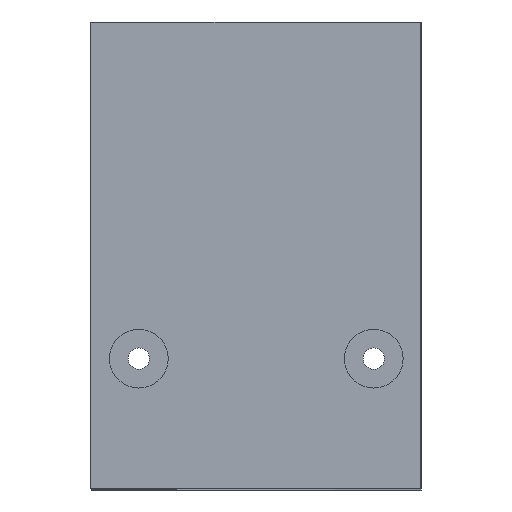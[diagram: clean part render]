
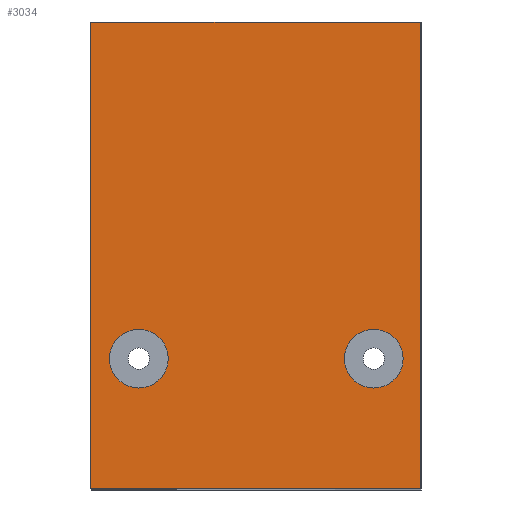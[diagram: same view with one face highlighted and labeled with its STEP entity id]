
A CAD part, front view. The second image highlights one B-rep face of the part: STEP entity #3034.
In plain terms, the highlighted planar face has unit normal (0, -1, 0).
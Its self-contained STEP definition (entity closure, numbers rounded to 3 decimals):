
#532 = PLANE('',#533);
#533 = AXIS2_PLACEMENT_3D('',#534,#535,#536);
#534 = CARTESIAN_POINT('',(76.2,22.676,20.811));
#535 = DIRECTION('',(0.,0.,-1.));
#536 = DIRECTION('',(0.,1.,0.));
#1657 = VERTEX_POINT('',#1658);
#1658 = CARTESIAN_POINT('',(76.103,23.345,20.811));
#1672 = PLANE('',#1673);
#1673 = AXIS2_PLACEMENT_3D('',#1674,#1675,#1676);
#1674 = CARTESIAN_POINT('',(76.103,42.545,-31.631));
#1675 = DIRECTION('',(-1.,0.,0.));
#1676 = DIRECTION('',(0.,0.,1.));
#1684 = EDGE_CURVE('',#1657,#1685,#1687,.T.);
#1685 = VERTEX_POINT('',#1686);
#1686 = CARTESIAN_POINT('',(39.094,23.345,20.811));
#1687 = SURFACE_CURVE('',#1688,(#1692,#1699),.PCURVE_S1.);
#1688 = LINE('',#1689,#1690);
#1689 = CARTESIAN_POINT('',(76.151,23.345,20.811));
#1690 = VECTOR('',#1691,1.);
#1691 = DIRECTION('',(-1.,0.,0.));
#1692 = PCURVE('',#532,#1693);
#1693 = DEFINITIONAL_REPRESENTATION('',(#1694),#1698);
#1694 = LINE('',#1695,#1696);
#1695 = CARTESIAN_POINT('',(0.669,-0.049));
#1696 = VECTOR('',#1697,1.);
#1697 = DIRECTION('',(0.,-1.));
#1698 = ( GEOMETRIC_REPRESENTATION_CONTEXT(2) 
PARAMETRIC_REPRESENTATION_CONTEXT() REPRESENTATION_CONTEXT('2D SPACE',''
  ) );
#1699 = PCURVE('',#1700,#1705);
#1700 = PLANE('',#1701);
#1701 = AXIS2_PLACEMENT_3D('',#1702,#1703,#1704);
#1702 = CARTESIAN_POINT('',(76.103,23.345,20.829));
#1703 = DIRECTION('',(0.,1.,0.));
#1704 = DIRECTION('',(0.,0.,1.));
#1705 = DEFINITIONAL_REPRESENTATION('',(#1706),#1710);
#1706 = LINE('',#1707,#1708);
#1707 = CARTESIAN_POINT('',(-0.018,0.049));
#1708 = VECTOR('',#1709,1.);
#1709 = DIRECTION('',(0.,-1.));
#1710 = ( GEOMETRIC_REPRESENTATION_CONTEXT(2) 
PARAMETRIC_REPRESENTATION_CONTEXT() REPRESENTATION_CONTEXT('2D SPACE',''
  ) );
#1726 = PLANE('',#1727);
#1727 = AXIS2_PLACEMENT_3D('',#1728,#1729,#1730);
#1728 = CARTESIAN_POINT('',(39.094,42.545,20.829));
#1729 = DIRECTION('',(1.,0.,0.));
#1730 = DIRECTION('',(0.,0.,-1.));
#1897 = PLANE('',#1898);
#1898 = AXIS2_PLACEMENT_3D('',#1899,#1900,#1901);
#1899 = CARTESIAN_POINT('',(39.094,42.545,-31.631));
#1900 = DIRECTION('',(0.,0.,1.));
#1901 = DIRECTION('',(1.,0.,0.));
#2990 = EDGE_CURVE('',#1685,#2991,#2993,.T.);
#2991 = VERTEX_POINT('',#2992);
#2992 = CARTESIAN_POINT('',(39.094,23.345,-31.631));
#2993 = SURFACE_CURVE('',#2994,(#2998,#3005),.PCURVE_S1.);
#2994 = LINE('',#2995,#2996);
#2995 = CARTESIAN_POINT('',(39.094,23.345,20.829));
#2996 = VECTOR('',#2997,1.);
#2997 = DIRECTION('',(0.,0.,-1.));
#2998 = PCURVE('',#1726,#2999);
#2999 = DEFINITIONAL_REPRESENTATION('',(#3000),#3004);
#3000 = LINE('',#3001,#3002);
#3001 = CARTESIAN_POINT('',(0.,-19.2));
#3002 = VECTOR('',#3003,1.);
#3003 = DIRECTION('',(1.,0.));
#3004 = ( GEOMETRIC_REPRESENTATION_CONTEXT(2) 
PARAMETRIC_REPRESENTATION_CONTEXT() REPRESENTATION_CONTEXT('2D SPACE',''
  ) );
#3005 = PCURVE('',#1700,#3006);
#3006 = DEFINITIONAL_REPRESENTATION('',(#3007),#3011);
#3007 = LINE('',#3008,#3009);
#3008 = CARTESIAN_POINT('',(0.,-37.009));
#3009 = VECTOR('',#3010,1.);
#3010 = DIRECTION('',(-1.,0.));
#3011 = ( GEOMETRIC_REPRESENTATION_CONTEXT(2) 
PARAMETRIC_REPRESENTATION_CONTEXT() REPRESENTATION_CONTEXT('2D SPACE',''
  ) );
#3034 = ADVANCED_FACE('',(#3035,#3083,#3118),#1700,.F.);
#3035 = FACE_BOUND('',#3036,.F.);
#3036 = EDGE_LOOP('',(#3037,#3038,#3061,#3082));
#3037 = ORIENTED_EDGE('',*,*,#1684,.F.);
#3038 = ORIENTED_EDGE('',*,*,#3039,.F.);
#3039 = EDGE_CURVE('',#3040,#1657,#3042,.T.);
#3040 = VERTEX_POINT('',#3041);
#3041 = CARTESIAN_POINT('',(76.103,23.345,-31.631));
#3042 = SURFACE_CURVE('',#3043,(#3047,#3054),.PCURVE_S1.);
#3043 = LINE('',#3044,#3045);
#3044 = CARTESIAN_POINT('',(76.103,23.345,-31.631));
#3045 = VECTOR('',#3046,1.);
#3046 = DIRECTION('',(0.,0.,1.));
#3047 = PCURVE('',#1700,#3048);
#3048 = DEFINITIONAL_REPRESENTATION('',(#3049),#3053);
#3049 = LINE('',#3050,#3051);
#3050 = CARTESIAN_POINT('',(-52.459,0.));
#3051 = VECTOR('',#3052,1.);
#3052 = DIRECTION('',(1.,0.));
#3053 = ( GEOMETRIC_REPRESENTATION_CONTEXT(2) 
PARAMETRIC_REPRESENTATION_CONTEXT() REPRESENTATION_CONTEXT('2D SPACE',''
  ) );
#3054 = PCURVE('',#1672,#3055);
#3055 = DEFINITIONAL_REPRESENTATION('',(#3056),#3060);
#3056 = LINE('',#3057,#3058);
#3057 = CARTESIAN_POINT('',(0.,-19.2));
#3058 = VECTOR('',#3059,1.);
#3059 = DIRECTION('',(1.,0.));
#3060 = ( GEOMETRIC_REPRESENTATION_CONTEXT(2) 
PARAMETRIC_REPRESENTATION_CONTEXT() REPRESENTATION_CONTEXT('2D SPACE',''
  ) );
#3061 = ORIENTED_EDGE('',*,*,#3062,.F.);
#3062 = EDGE_CURVE('',#2991,#3040,#3063,.T.);
#3063 = SURFACE_CURVE('',#3064,(#3068,#3075),.PCURVE_S1.);
#3064 = LINE('',#3065,#3066);
#3065 = CARTESIAN_POINT('',(39.094,23.345,-31.631));
#3066 = VECTOR('',#3067,1.);
#3067 = DIRECTION('',(1.,0.,0.));
#3068 = PCURVE('',#1700,#3069);
#3069 = DEFINITIONAL_REPRESENTATION('',(#3070),#3074);
#3070 = LINE('',#3071,#3072);
#3071 = CARTESIAN_POINT('',(-52.459,-37.009));
#3072 = VECTOR('',#3073,1.);
#3073 = DIRECTION('',(0.,1.));
#3074 = ( GEOMETRIC_REPRESENTATION_CONTEXT(2) 
PARAMETRIC_REPRESENTATION_CONTEXT() REPRESENTATION_CONTEXT('2D SPACE',''
  ) );
#3075 = PCURVE('',#1897,#3076);
#3076 = DEFINITIONAL_REPRESENTATION('',(#3077),#3081);
#3077 = LINE('',#3078,#3079);
#3078 = CARTESIAN_POINT('',(0.,-19.2));
#3079 = VECTOR('',#3080,1.);
#3080 = DIRECTION('',(1.,0.));
#3081 = ( GEOMETRIC_REPRESENTATION_CONTEXT(2) 
PARAMETRIC_REPRESENTATION_CONTEXT() REPRESENTATION_CONTEXT('2D SPACE',''
  ) );
#3082 = ORIENTED_EDGE('',*,*,#2990,.F.);
#3083 = FACE_BOUND('',#3084,.F.);
#3084 = EDGE_LOOP('',(#3085));
#3085 = ORIENTED_EDGE('',*,*,#3086,.T.);
#3086 = EDGE_CURVE('',#3087,#3087,#3089,.T.);
#3087 = VERTEX_POINT('',#3088);
#3088 = CARTESIAN_POINT('',(47.792,23.345,-17.));
#3089 = SURFACE_CURVE('',#3090,(#3095,#3106),.PCURVE_S1.);
#3090 = CIRCLE('',#3091,3.3);
#3091 = AXIS2_PLACEMENT_3D('',#3092,#3093,#3094);
#3092 = CARTESIAN_POINT('',(44.492,23.345,-17.));
#3093 = DIRECTION('',(0.,-1.,0.));
#3094 = DIRECTION('',(1.,0.,0.));
#3095 = PCURVE('',#1700,#3096);
#3096 = DEFINITIONAL_REPRESENTATION('',(#3097),#3105);
#3097 = ( BOUNDED_CURVE() B_SPLINE_CURVE(2,(#3098,#3099,#3100,#3101,
#3102,#3103,#3104),.UNSPECIFIED.,.T.,.F.) B_SPLINE_CURVE_WITH_KNOTS((1,2
    ,2,2,2,1),(-2.094,0.,2.094,4.189,
6.283,8.378),.UNSPECIFIED.) CURVE() 
GEOMETRIC_REPRESENTATION_ITEM() RATIONAL_B_SPLINE_CURVE((1.,0.5,1.,0.5,
1.,0.5,1.)) REPRESENTATION_ITEM('') );
#3098 = CARTESIAN_POINT('',(-37.829,-28.31));
#3099 = CARTESIAN_POINT('',(-32.113,-28.31));
#3100 = CARTESIAN_POINT('',(-34.971,-33.26));
#3101 = CARTESIAN_POINT('',(-37.829,-38.21));
#3102 = CARTESIAN_POINT('',(-40.686,-33.26));
#3103 = CARTESIAN_POINT('',(-43.544,-28.31));
#3104 = CARTESIAN_POINT('',(-37.829,-28.31));
#3105 = ( GEOMETRIC_REPRESENTATION_CONTEXT(2) 
PARAMETRIC_REPRESENTATION_CONTEXT() REPRESENTATION_CONTEXT('2D SPACE',''
  ) );
#3106 = PCURVE('',#3107,#3112);
#3107 = CYLINDRICAL_SURFACE('',#3108,3.3);
#3108 = AXIS2_PLACEMENT_3D('',#3109,#3110,#3111);
#3109 = CARTESIAN_POINT('',(44.492,23.345,-17.));
#3110 = DIRECTION('',(0.,-1.,0.));
#3111 = DIRECTION('',(1.,0.,0.));
#3112 = DEFINITIONAL_REPRESENTATION('',(#3113),#3117);
#3113 = LINE('',#3114,#3115);
#3114 = CARTESIAN_POINT('',(0.,0.));
#3115 = VECTOR('',#3116,1.);
#3116 = DIRECTION('',(1.,0.));
#3117 = ( GEOMETRIC_REPRESENTATION_CONTEXT(2) 
PARAMETRIC_REPRESENTATION_CONTEXT() REPRESENTATION_CONTEXT('2D SPACE',''
  ) );
#3118 = FACE_BOUND('',#3119,.F.);
#3119 = EDGE_LOOP('',(#3120));
#3120 = ORIENTED_EDGE('',*,*,#3121,.T.);
#3121 = EDGE_CURVE('',#3122,#3122,#3124,.T.);
#3122 = VERTEX_POINT('',#3123);
#3123 = CARTESIAN_POINT('',(74.175,23.345,-17.));
#3124 = SURFACE_CURVE('',#3125,(#3130,#3141),.PCURVE_S1.);
#3125 = CIRCLE('',#3126,3.3);
#3126 = AXIS2_PLACEMENT_3D('',#3127,#3128,#3129);
#3127 = CARTESIAN_POINT('',(70.875,23.345,-17.));
#3128 = DIRECTION('',(0.,-1.,0.));
#3129 = DIRECTION('',(1.,0.,0.));
#3130 = PCURVE('',#1700,#3131);
#3131 = DEFINITIONAL_REPRESENTATION('',(#3132),#3140);
#3132 = ( BOUNDED_CURVE() B_SPLINE_CURVE(2,(#3133,#3134,#3135,#3136,
#3137,#3138,#3139),.UNSPECIFIED.,.T.,.F.) B_SPLINE_CURVE_WITH_KNOTS((1,2
    ,2,2,2,1),(-2.094,0.,2.094,4.189,
6.283,8.378),.UNSPECIFIED.) CURVE() 
GEOMETRIC_REPRESENTATION_ITEM() RATIONAL_B_SPLINE_CURVE((1.,0.5,1.,0.5,
1.,0.5,1.)) REPRESENTATION_ITEM('') );
#3133 = CARTESIAN_POINT('',(-37.829,-1.927));
#3134 = CARTESIAN_POINT('',(-32.113,-1.927));
#3135 = CARTESIAN_POINT('',(-34.971,-6.877));
#3136 = CARTESIAN_POINT('',(-37.829,-11.827));
#3137 = CARTESIAN_POINT('',(-40.686,-6.877));
#3138 = CARTESIAN_POINT('',(-43.544,-1.927));
#3139 = CARTESIAN_POINT('',(-37.829,-1.927));
#3140 = ( GEOMETRIC_REPRESENTATION_CONTEXT(2) 
PARAMETRIC_REPRESENTATION_CONTEXT() REPRESENTATION_CONTEXT('2D SPACE',''
  ) );
#3141 = PCURVE('',#3142,#3147);
#3142 = CYLINDRICAL_SURFACE('',#3143,3.3);
#3143 = AXIS2_PLACEMENT_3D('',#3144,#3145,#3146);
#3144 = CARTESIAN_POINT('',(70.875,23.345,-17.));
#3145 = DIRECTION('',(0.,-1.,0.));
#3146 = DIRECTION('',(1.,0.,0.));
#3147 = DEFINITIONAL_REPRESENTATION('',(#3148),#3152);
#3148 = LINE('',#3149,#3150);
#3149 = CARTESIAN_POINT('',(0.,0.));
#3150 = VECTOR('',#3151,1.);
#3151 = DIRECTION('',(1.,0.));
#3152 = ( GEOMETRIC_REPRESENTATION_CONTEXT(2) 
PARAMETRIC_REPRESENTATION_CONTEXT() REPRESENTATION_CONTEXT('2D SPACE',''
  ) );
